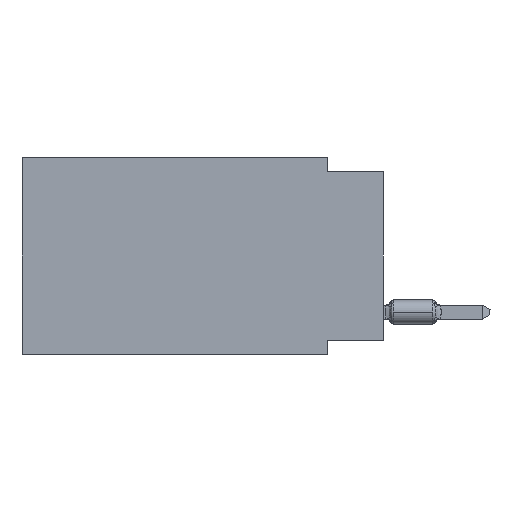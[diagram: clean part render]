
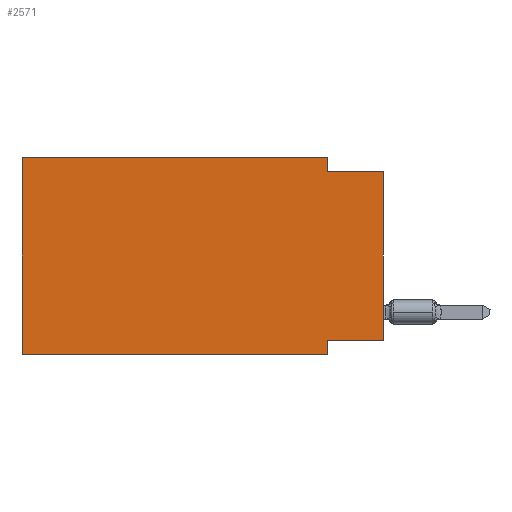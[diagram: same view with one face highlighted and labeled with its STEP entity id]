
A CAD part, left-side view. The second image highlights one B-rep face of the part: STEP entity #2571.
In plain terms, the highlighted planar face has unit normal (-1, 0, 0).
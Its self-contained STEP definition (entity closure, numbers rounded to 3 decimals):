
#431 = VECTOR ( 'NONE', #1875, 1000. ) ;
#1537 = DIRECTION ( 'NONE',  ( 0., 0., -1. ) ) ;
#1875 = DIRECTION ( 'NONE',  ( 0., 0., -1. ) ) ;
#1926 = ORIENTED_EDGE ( 'NONE', *, *, #67488, .F. ) ;
#2201 = LINE ( 'NONE', #44203, #33996 ) ;
#2281 = DIRECTION ( 'NONE',  ( 0., 1., 0. ) ) ;
#2429 = CARTESIAN_POINT ( 'NONE',  ( 0., 0., -0.635 ) ) ;
#2571 = ADVANCED_FACE ( 'NONE', ( #4680 ), #36183, .F. ) ;
#3020 = EDGE_CURVE ( 'NONE', #26625, #18730, #13377, .T. ) ;
#3806 = DIRECTION ( 'NONE',  ( 0., -1., 0. ) ) ;
#4680 = FACE_OUTER_BOUND ( 'NONE', #60022, .T. ) ;
#9072 = CARTESIAN_POINT ( 'NONE',  ( 0., 2.54, -0.635 ) ) ;
#12886 = ORIENTED_EDGE ( 'NONE', *, *, #46775, .F. ) ;
#13377 = LINE ( 'NONE', #62987, #66981 ) ;
#13910 = VECTOR ( 'NONE', #1537, 1000. ) ;
#14007 = LINE ( 'NONE', #35365, #51998 ) ;
#14141 = CARTESIAN_POINT ( 'NONE',  ( 0., 16.383, 0. ) ) ;
#18072 = LINE ( 'NONE', #45005, #60929 ) ;
#18470 = VERTEX_POINT ( 'NONE', #45036 ) ;
#18730 = VERTEX_POINT ( 'NONE', #47473 ) ;
#19386 = CARTESIAN_POINT ( 'NONE',  ( 0., 0., -8.255 ) ) ;
#20083 = DIRECTION ( 'NONE',  ( 0., 0., -1. ) ) ;
#22424 = ORIENTED_EDGE ( 'NONE', *, *, #47633, .F. ) ;
#23357 = EDGE_CURVE ( 'NONE', #36388, #34584, #33049, .T. ) ;
#24637 = DIRECTION ( 'NONE',  ( 1., 0., 0. ) ) ;
#24973 = EDGE_CURVE ( 'NONE', #63092, #36388, #14007, .T. ) ;
#25610 = DIRECTION ( 'NONE',  ( 0., -1., 0. ) ) ;
#26625 = VERTEX_POINT ( 'NONE', #56606 ) ;
#28542 = LINE ( 'NONE', #19386, #54025 ) ;
#29422 = DIRECTION ( 'NONE',  ( 0., -1., 0. ) ) ;
#31312 = CARTESIAN_POINT ( 'NONE',  ( 0., 0., -0.635 ) ) ;
#32776 = ORIENTED_EDGE ( 'NONE', *, *, #36334, .T. ) ;
#33049 = LINE ( 'NONE', #60277, #431 ) ;
#33996 = VECTOR ( 'NONE', #45216, 1000. ) ;
#34227 = ORIENTED_EDGE ( 'NONE', *, *, #3020, .T. ) ;
#34584 = VERTEX_POINT ( 'NONE', #9072 ) ;
#34779 = CARTESIAN_POINT ( 'NONE',  ( 0., 2.54, -8.89 ) ) ;
#35365 = CARTESIAN_POINT ( 'NONE',  ( 0., 16.383, 0. ) ) ;
#36183 = PLANE ( 'NONE',  #69197 ) ;
#36334 = EDGE_CURVE ( 'NONE', #18470, #57463, #2201, .T. ) ;
#36388 = VERTEX_POINT ( 'NONE', #66534 ) ;
#39426 = DIRECTION ( 'NONE',  ( 0., 0., 1. ) ) ;
#41606 = VECTOR ( 'NONE', #3806, 1000. ) ;
#42506 = ORIENTED_EDGE ( 'NONE', *, *, #23357, .F. ) ;
#43671 = EDGE_CURVE ( 'NONE', #34584, #57463, #51733, .T. ) ;
#44203 = CARTESIAN_POINT ( 'NONE',  ( 0., 0., 0. ) ) ;
#44246 = LINE ( 'NONE', #34779, #13910 ) ;
#45005 = CARTESIAN_POINT ( 'NONE',  ( 0., 16.383, 0. ) ) ;
#45036 = CARTESIAN_POINT ( 'NONE',  ( 0., 0., -8.255 ) ) ;
#45216 = DIRECTION ( 'NONE',  ( 0., 0., 1. ) ) ;
#46775 = EDGE_CURVE ( 'NONE', #62640, #18730, #44246, .T. ) ;
#47473 = CARTESIAN_POINT ( 'NONE',  ( 0., 2.54, -8.89 ) ) ;
#47633 = EDGE_CURVE ( 'NONE', #26625, #63092, #18072, .T. ) ;
#51733 = LINE ( 'NONE', #2429, #41606 ) ;
#51998 = VECTOR ( 'NONE', #29422, 1000. ) ;
#54025 = VECTOR ( 'NONE', #2281, 1000. ) ;
#56606 = CARTESIAN_POINT ( 'NONE',  ( 0., 16.383, -8.89 ) ) ;
#57463 = VERTEX_POINT ( 'NONE', #31312 ) ;
#60022 = EDGE_LOOP ( 'NONE', ( #32776, #68068, #42506, #65834, #22424, #34227, #12886, #1926 ) ) ;
#60187 = CARTESIAN_POINT ( 'NONE',  ( 0., 16.383, 0. ) ) ;
#60277 = CARTESIAN_POINT ( 'NONE',  ( 0., 2.54, 0. ) ) ;
#60929 = VECTOR ( 'NONE', #39426, 1000. ) ;
#62483 = CARTESIAN_POINT ( 'NONE',  ( 0., 2.54, -8.255 ) ) ;
#62640 = VERTEX_POINT ( 'NONE', #62483 ) ;
#62987 = CARTESIAN_POINT ( 'NONE',  ( 0., 16.383, -8.89 ) ) ;
#63092 = VERTEX_POINT ( 'NONE', #60187 ) ;
#65834 = ORIENTED_EDGE ( 'NONE', *, *, #24973, .F. ) ;
#66534 = CARTESIAN_POINT ( 'NONE',  ( 0., 2.54, 0. ) ) ;
#66981 = VECTOR ( 'NONE', #25610, 1000. ) ;
#67488 = EDGE_CURVE ( 'NONE', #18470, #62640, #28542, .T. ) ;
#68068 = ORIENTED_EDGE ( 'NONE', *, *, #43671, .F. ) ;
#69197 = AXIS2_PLACEMENT_3D ( 'NONE', #14141, #24637, #20083 ) ;
